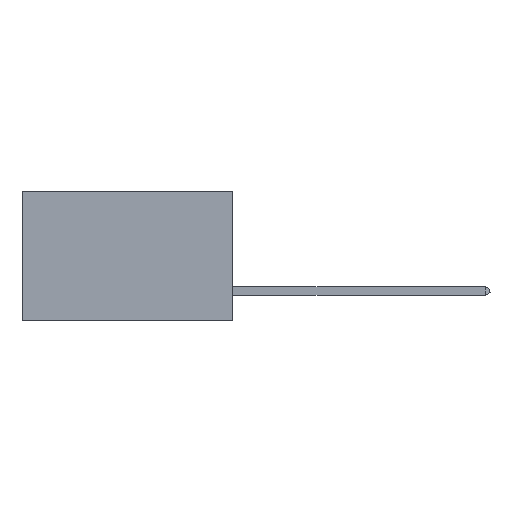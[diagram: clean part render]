
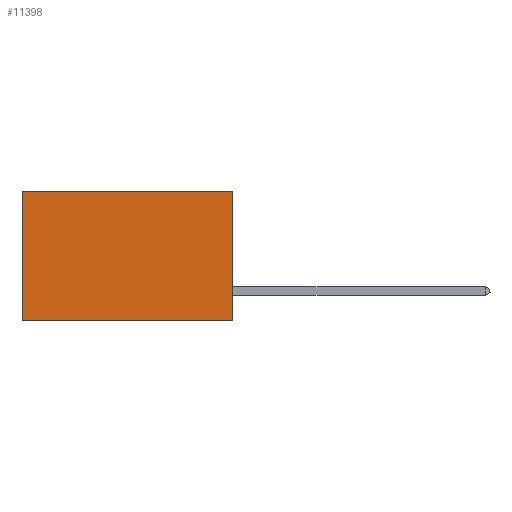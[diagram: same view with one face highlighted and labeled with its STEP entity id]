
A CAD part, left-side view. The second image highlights one B-rep face of the part: STEP entity #11398.
In plain terms, the highlighted planar face has unit normal (-1, 0, 0).
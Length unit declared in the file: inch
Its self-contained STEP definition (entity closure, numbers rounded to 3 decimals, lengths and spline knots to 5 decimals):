
#1044 = LINE ( 'NONE', #1432, #16655 ) ;
#1360 = EDGE_CURVE ( 'NONE', #8370, #8354, #4637, .T. ) ;
#1432 = CARTESIAN_POINT ( 'NONE',  ( 0.2875, 0., 0. ) ) ;
#1630 = VECTOR ( 'NONE', #7660, 39.37008 ) ;
#1653 = CARTESIAN_POINT ( 'NONE',  ( 0.2875, 0., -0.37 ) ) ;
#2411 = VERTEX_POINT ( 'NONE', #9361 ) ;
#2686 = PLANE ( 'NONE',  #19252 ) ;
#2708 = EDGE_CURVE ( 'NONE', #8370, #13639, #1044, .T. ) ;
#3702 = VECTOR ( 'NONE', #18823, 39.37008 ) ;
#4471 = EDGE_CURVE ( 'NONE', #13639, #2411, #16123, .T. ) ;
#4637 = LINE ( 'NONE', #12662, #3702 ) ;
#5182 = ORIENTED_EDGE ( 'NONE', *, *, #4471, .T. ) ;
#5544 = CARTESIAN_POINT ( 'NONE',  ( 0.2875, 0., 0. ) ) ;
#5678 = LINE ( 'NONE', #1653, #1630 ) ;
#5763 = FACE_OUTER_BOUND ( 'NONE', #12261, .T. ) ;
#6334 = CARTESIAN_POINT ( 'NONE',  ( 0.2875, 0.6, 0. ) ) ;
#7660 = DIRECTION ( 'NONE',  ( 0., 1., 0. ) ) ;
#7697 = CARTESIAN_POINT ( 'NONE',  ( 0.2875, 0.6, 0. ) ) ;
#8117 = VECTOR ( 'NONE', #14070, 39.37008 ) ;
#8354 = VERTEX_POINT ( 'NONE', #16029 ) ;
#8370 = VERTEX_POINT ( 'NONE', #5544 ) ;
#8689 = EDGE_CURVE ( 'NONE', #8354, #2411, #5678, .T. ) ;
#9361 = CARTESIAN_POINT ( 'NONE',  ( 0.2875, 0.6, -0.37 ) ) ;
#10081 = ORIENTED_EDGE ( 'NONE', *, *, #2708, .T. ) ;
#10300 = DIRECTION ( 'NONE',  ( 1., 0., 0. ) ) ;
#10361 = DIRECTION ( 'NONE',  ( 0., 0., -1. ) ) ;
#10773 = ORIENTED_EDGE ( 'NONE', *, *, #1360, .F. ) ;
#11398 = ADVANCED_FACE ( 'NONE', ( #5763 ), #2686, .F. ) ;
#12186 = ORIENTED_EDGE ( 'NONE', *, *, #8689, .F. ) ;
#12261 = EDGE_LOOP ( 'NONE', ( #5182, #12186, #10773, #10081 ) ) ;
#12662 = CARTESIAN_POINT ( 'NONE',  ( 0.2875, 0., 0. ) ) ;
#13339 = DIRECTION ( 'NONE',  ( 0., 1., 0. ) ) ;
#13639 = VERTEX_POINT ( 'NONE', #7697 ) ;
#14070 = DIRECTION ( 'NONE',  ( 0., 0., -1. ) ) ;
#16029 = CARTESIAN_POINT ( 'NONE',  ( 0.2875, 0., -0.37 ) ) ;
#16123 = LINE ( 'NONE', #6334, #8117 ) ;
#16324 = CARTESIAN_POINT ( 'NONE',  ( 0.2875, 0., 0. ) ) ;
#16655 = VECTOR ( 'NONE', #13339, 39.37008 ) ;
#18823 = DIRECTION ( 'NONE',  ( 0., 0., -1. ) ) ;
#19252 = AXIS2_PLACEMENT_3D ( 'NONE', #16324, #10300, #10361 ) ;
